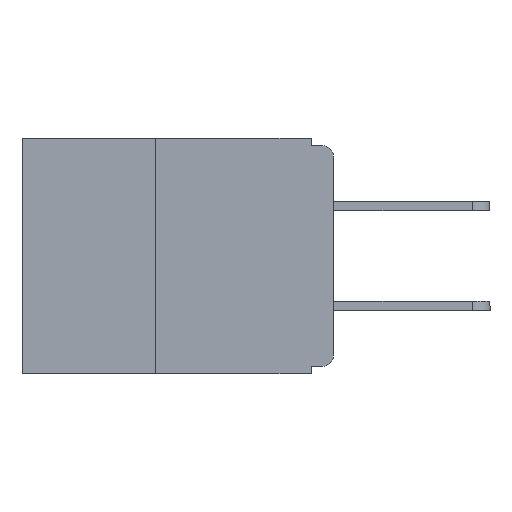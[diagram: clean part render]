
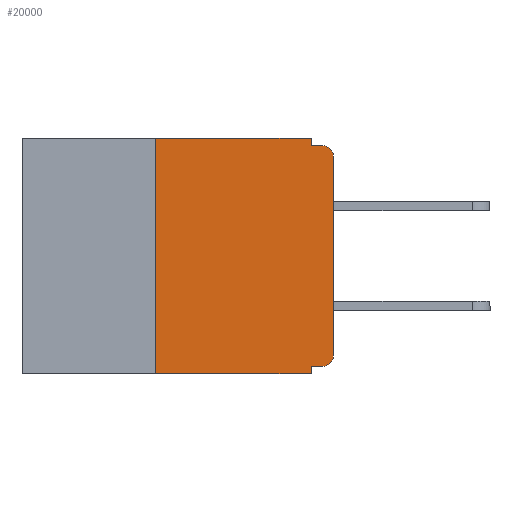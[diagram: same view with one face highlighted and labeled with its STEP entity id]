
A CAD part, left-side view. The second image highlights one B-rep face of the part: STEP entity #20000.
In plain terms, the highlighted planar face has unit normal (-1, 0, 0).
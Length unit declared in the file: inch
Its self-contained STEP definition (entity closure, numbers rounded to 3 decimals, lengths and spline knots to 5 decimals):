
#606 = CARTESIAN_POINT ( 'NONE',  ( 0., 0., -0.025 ) ) ;
#1079 = DIRECTION ( 'NONE',  ( 0., 0., 1. ) ) ;
#2083 = ORIENTED_EDGE ( 'NONE', *, *, #8066, .F. ) ;
#2088 = DIRECTION ( 'NONE',  ( -1., 0., 0. ) ) ;
#2138 = LINE ( 'NONE', #5054, #2703 ) ;
#2186 = AXIS2_PLACEMENT_3D ( 'NONE', #3548, #3538, #3471 ) ;
#2206 = LINE ( 'NONE', #2695, #15252 ) ;
#2695 = CARTESIAN_POINT ( 'NONE',  ( 0., 0.437, -0.33 ) ) ;
#2703 = VECTOR ( 'NONE', #6799, 39.37008 ) ;
#2880 = DIRECTION ( 'NONE',  ( 0., 0., -1. ) ) ;
#2900 = VERTEX_POINT ( 'NONE', #6292 ) ;
#2946 = VECTOR ( 'NONE', #1079, 39.37008 ) ;
#2980 = ORIENTED_EDGE ( 'NONE', *, *, #17977, .T. ) ;
#3301 = EDGE_CURVE ( 'NONE', #14655, #2900, #15136, .T. ) ;
#3471 = DIRECTION ( 'NONE',  ( 0., 0., -1. ) ) ;
#3538 = DIRECTION ( 'NONE',  ( -1., 0., 0. ) ) ;
#3548 = CARTESIAN_POINT ( 'NONE',  ( 0., 0.015, -0.025 ) ) ;
#3564 = VERTEX_POINT ( 'NONE', #15694 ) ;
#3939 = LINE ( 'NONE', #19619, #8493 ) ;
#4098 = VECTOR ( 'NONE', #16512, 39.37008 ) ;
#4321 = ORIENTED_EDGE ( 'NONE', *, *, #19764, .T. ) ;
#4475 = DIRECTION ( 'NONE',  ( 0., -1., 0. ) ) ;
#4820 = VERTEX_POINT ( 'NONE', #7685 ) ;
#4841 = DIRECTION ( 'NONE',  ( 0., 1., 0. ) ) ;
#4843 = ORIENTED_EDGE ( 'NONE', *, *, #18236, .F. ) ;
#5054 = CARTESIAN_POINT ( 'NONE',  ( 0., 0., -0.01 ) ) ;
#5252 = CIRCLE ( 'NONE', #14309, 0.015 ) ;
#5446 = VERTEX_POINT ( 'NONE', #11388 ) ;
#5617 = ORIENTED_EDGE ( 'NONE', *, *, #3301, .T. ) ;
#5986 = LINE ( 'NONE', #21214, #10013 ) ;
#6235 = CARTESIAN_POINT ( 'NONE',  ( 0., 0.015, -0.32 ) ) ;
#6292 = CARTESIAN_POINT ( 'NONE',  ( 0., 0.015, -0.01 ) ) ;
#6770 = DIRECTION ( 'NONE',  ( 1., 0., 0. ) ) ;
#6799 = DIRECTION ( 'NONE',  ( 0., -1., 0. ) ) ;
#7685 = CARTESIAN_POINT ( 'NONE',  ( 0., 0., -0.305 ) ) ;
#8066 = EDGE_CURVE ( 'NONE', #20297, #9937, #5986, .T. ) ;
#8438 = CARTESIAN_POINT ( 'NONE',  ( 0., 0.031, -0.33 ) ) ;
#8493 = VECTOR ( 'NONE', #2880, 39.37008 ) ;
#8889 = CARTESIAN_POINT ( 'NONE',  ( 0., 0.25, -0.33 ) ) ;
#9139 = DIRECTION ( 'NONE',  ( 0., -1., 0. ) ) ;
#9173 = LINE ( 'NONE', #21331, #4098 ) ;
#9660 = DIRECTION ( 'NONE',  ( 0., 0., -1. ) ) ;
#9717 = VECTOR ( 'NONE', #9139, 39.37008 ) ;
#9937 = VERTEX_POINT ( 'NONE', #19587 ) ;
#10013 = VECTOR ( 'NONE', #9660, 39.37008 ) ;
#10359 = VECTOR ( 'NONE', #4841, 39.37008 ) ;
#11032 = CARTESIAN_POINT ( 'NONE',  ( 0., 0.031, 0. ) ) ;
#11107 = FACE_OUTER_BOUND ( 'NONE', #21422, .T. ) ;
#11305 = EDGE_CURVE ( 'NONE', #5446, #20297, #14197, .T. ) ;
#11388 = CARTESIAN_POINT ( 'NONE',  ( 0., 0.25, 0. ) ) ;
#11681 = CARTESIAN_POINT ( 'NONE',  ( 0., 0., -0.32 ) ) ;
#11690 = EDGE_CURVE ( 'NONE', #9937, #2900, #2138, .T. ) ;
#12313 = ORIENTED_EDGE ( 'NONE', *, *, #11305, .F. ) ;
#12394 = CARTESIAN_POINT ( 'NONE',  ( 0., 0.015, -0.305 ) ) ;
#12747 = EDGE_CURVE ( 'NONE', #4820, #14655, #16459, .T. ) ;
#14057 = DIRECTION ( 'NONE',  ( 0., 0., -1. ) ) ;
#14140 = CARTESIAN_POINT ( 'NONE',  ( 0., 0.437, 0. ) ) ;
#14197 = LINE ( 'NONE', #14140, #9717 ) ;
#14309 = AXIS2_PLACEMENT_3D ( 'NONE', #12394, #2088, #14057 ) ;
#14655 = VERTEX_POINT ( 'NONE', #606 ) ;
#14794 = LINE ( 'NONE', #11681, #10359 ) ;
#15101 = PLANE ( 'NONE',  #19115 ) ;
#15136 = CIRCLE ( 'NONE', #2186, 0.015 ) ;
#15252 = VECTOR ( 'NONE', #4475, 39.37008 ) ;
#15694 = CARTESIAN_POINT ( 'NONE',  ( 0., 0.031, -0.32 ) ) ;
#15942 = ORIENTED_EDGE ( 'NONE', *, *, #18335, .F. ) ;
#16459 = LINE ( 'NONE', #21282, #2946 ) ;
#16512 = DIRECTION ( 'NONE',  ( 0., 0., 1. ) ) ;
#16699 = VERTEX_POINT ( 'NONE', #8889 ) ;
#16713 = ORIENTED_EDGE ( 'NONE', *, *, #21142, .F. ) ;
#16840 = CARTESIAN_POINT ( 'NONE',  ( 0., 0.437, 0. ) ) ;
#17977 = EDGE_CURVE ( 'NONE', #18888, #4820, #5252, .T. ) ;
#18236 = EDGE_CURVE ( 'NONE', #3564, #19986, #3939, .T. ) ;
#18335 = EDGE_CURVE ( 'NONE', #18888, #3564, #14794, .T. ) ;
#18454 = DIRECTION ( 'NONE',  ( 0., 0., -1. ) ) ;
#18888 = VERTEX_POINT ( 'NONE', #6235 ) ;
#19115 = AXIS2_PLACEMENT_3D ( 'NONE', #16840, #6770, #18454 ) ;
#19219 = ORIENTED_EDGE ( 'NONE', *, *, #12747, .T. ) ;
#19493 = ORIENTED_EDGE ( 'NONE', *, *, #11690, .F. ) ;
#19587 = CARTESIAN_POINT ( 'NONE',  ( 0., 0.031, -0.01 ) ) ;
#19619 = CARTESIAN_POINT ( 'NONE',  ( 0., 0.031, -0.33 ) ) ;
#19764 = EDGE_CURVE ( 'NONE', #16699, #19986, #2206, .T. ) ;
#19986 = VERTEX_POINT ( 'NONE', #8438 ) ;
#20000 = ADVANCED_FACE ( 'NONE', ( #11107 ), #15101, .F. ) ;
#20297 = VERTEX_POINT ( 'NONE', #11032 ) ;
#21142 = EDGE_CURVE ( 'NONE', #16699, #5446, #9173, .T. ) ;
#21214 = CARTESIAN_POINT ( 'NONE',  ( 0., 0.031, 0. ) ) ;
#21282 = CARTESIAN_POINT ( 'NONE',  ( 0., 0., 0. ) ) ;
#21331 = CARTESIAN_POINT ( 'NONE',  ( 0., 0.25, -0.33 ) ) ;
#21422 = EDGE_LOOP ( 'NONE', ( #19219, #5617, #19493, #2083, #12313, #16713, #4321, #4843, #15942, #2980 ) ) ;
